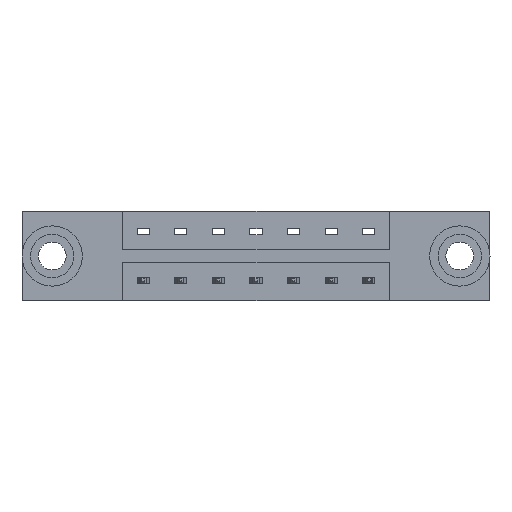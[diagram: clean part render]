
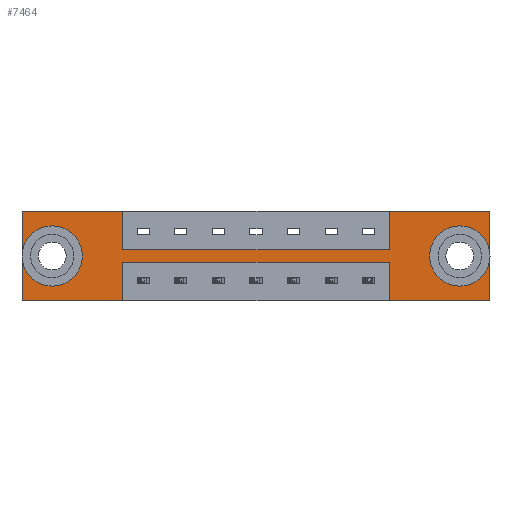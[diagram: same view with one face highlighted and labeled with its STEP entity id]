
A CAD part, front view. The second image highlights one B-rep face of the part: STEP entity #7464.
In plain terms, the highlighted planar face has unit normal (0, -1, 0).
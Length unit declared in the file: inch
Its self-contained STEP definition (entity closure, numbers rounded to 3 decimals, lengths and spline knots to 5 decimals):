
#50 = DIRECTION ( 'NONE',  ( 0., 0., 1. ) ) ;
#335 = CARTESIAN_POINT ( 'NONE',  ( 1.94, 0., 0. ) ) ;
#373 = ORIENTED_EDGE ( 'NONE', *, *, #9041, .F. ) ;
#390 = CARTESIAN_POINT ( 'NONE',  ( 0.4175, 0., -0.2115 ) ) ;
#518 = CARTESIAN_POINT ( 'NONE',  ( 1.5225, 0., -0.37 ) ) ;
#649 = AXIS2_PLACEMENT_3D ( 'NONE', #8227, #1374, #8664 ) ;
#770 = CARTESIAN_POINT ( 'NONE',  ( 1.5225, 0., -0.1585 ) ) ;
#817 = CIRCLE ( 'NONE', #2033, 0.078 ) ;
#856 = EDGE_CURVE ( 'NONE', #5274, #5009, #817, .T. ) ;
#886 = LINE ( 'NONE', #2596, #6320 ) ;
#990 = DIRECTION ( 'NONE',  ( 0., 0., -1. ) ) ;
#1005 = DIRECTION ( 'NONE',  ( 0., 0., 1. ) ) ;
#1165 = EDGE_CURVE ( 'NONE', #5626, #3667, #4683, .T. ) ;
#1167 = VERTEX_POINT ( 'NONE', #4730 ) ;
#1338 = VERTEX_POINT ( 'NONE', #4372 ) ;
#1363 = CARTESIAN_POINT ( 'NONE',  ( 1.815, 0., -0.185 ) ) ;
#1374 = DIRECTION ( 'NONE',  ( 0., 1., 0. ) ) ;
#1428 = DIRECTION ( 'NONE',  ( 0., 1., 0. ) ) ;
#1443 = VECTOR ( 'NONE', #990, 39.37008 ) ;
#1473 = VECTOR ( 'NONE', #3516, 39.37008 ) ;
#1480 = ORIENTED_EDGE ( 'NONE', *, *, #3855, .F. ) ;
#1493 = CARTESIAN_POINT ( 'NONE',  ( 1.94, 0., -0.37 ) ) ;
#1582 = CIRCLE ( 'NONE', #6945, 0.078 ) ;
#1645 = DIRECTION ( 'NONE',  ( 0., 0., 1. ) ) ;
#1690 = ORIENTED_EDGE ( 'NONE', *, *, #4533, .F. ) ;
#1694 = CARTESIAN_POINT ( 'NONE',  ( 0., 0., 0. ) ) ;
#1730 = FACE_BOUND ( 'NONE', #6455, .T. ) ;
#1777 = DIRECTION ( 'NONE',  ( -1., 0., 0. ) ) ;
#1828 = CARTESIAN_POINT ( 'NONE',  ( 0., 0., -0.37 ) ) ;
#1865 = DIRECTION ( 'NONE',  ( 0., -1., 0. ) ) ;
#1925 = DIRECTION ( 'NONE',  ( 1., 0., 0. ) ) ;
#1954 = EDGE_CURVE ( 'NONE', #8772, #3220, #3174, .T. ) ;
#2033 = AXIS2_PLACEMENT_3D ( 'NONE', #1363, #9316, #5022 ) ;
#2048 = VECTOR ( 'NONE', #1005, 39.37008 ) ;
#2087 = ORIENTED_EDGE ( 'NONE', *, *, #4001, .T. ) ;
#2151 = CARTESIAN_POINT ( 'NONE',  ( 0., 0., -0.37 ) ) ;
#2207 = CARTESIAN_POINT ( 'NONE',  ( 0.4175, 0., -0.2115 ) ) ;
#2354 = VECTOR ( 'NONE', #3242, 39.37008 ) ;
#2374 = CARTESIAN_POINT ( 'NONE',  ( 0.4175, 0., -0.1585 ) ) ;
#2454 = VERTEX_POINT ( 'NONE', #1493 ) ;
#2457 = CARTESIAN_POINT ( 'NONE',  ( 0.4175, 0., -0.37 ) ) ;
#2596 = CARTESIAN_POINT ( 'NONE',  ( 0., 0., 0. ) ) ;
#2638 = LINE ( 'NONE', #5570, #4500 ) ;
#2651 = LINE ( 'NONE', #335, #3475 ) ;
#2691 = ORIENTED_EDGE ( 'NONE', *, *, #1165, .F. ) ;
#2781 = CARTESIAN_POINT ( 'NONE',  ( 1.5225, 0., -0.1585 ) ) ;
#2901 = CARTESIAN_POINT ( 'NONE',  ( 1.5225, 0., 0. ) ) ;
#2927 = CARTESIAN_POINT ( 'NONE',  ( 0.125, 0., -0.185 ) ) ;
#2931 = LINE ( 'NONE', #2207, #5883 ) ;
#3144 = EDGE_CURVE ( 'NONE', #8902, #3191, #3716, .T. ) ;
#3174 = LINE ( 'NONE', #4558, #1443 ) ;
#3191 = VERTEX_POINT ( 'NONE', #6732 ) ;
#3220 = VERTEX_POINT ( 'NONE', #2374 ) ;
#3242 = DIRECTION ( 'NONE',  ( 0., 0., -1. ) ) ;
#3268 = CARTESIAN_POINT ( 'NONE',  ( 0., 0., -0.37 ) ) ;
#3282 = CARTESIAN_POINT ( 'NONE',  ( 0., 0., -0.37 ) ) ;
#3327 = ORIENTED_EDGE ( 'NONE', *, *, #7932, .F. ) ;
#3335 = DIRECTION ( 'NONE',  ( 0., 0., -1. ) ) ;
#3475 = VECTOR ( 'NONE', #5580, 39.37008 ) ;
#3516 = DIRECTION ( 'NONE',  ( 0., 0., 1. ) ) ;
#3526 = VERTEX_POINT ( 'NONE', #770 ) ;
#3595 = VECTOR ( 'NONE', #1777, 39.37008 ) ;
#3667 = VERTEX_POINT ( 'NONE', #2457 ) ;
#3716 = LINE ( 'NONE', #8886, #6214 ) ;
#3739 = ORIENTED_EDGE ( 'NONE', *, *, #856, .T. ) ;
#3813 = VERTEX_POINT ( 'NONE', #6146 ) ;
#3855 = EDGE_CURVE ( 'NONE', #3526, #4799, #9338, .T. ) ;
#3961 = DIRECTION ( 'NONE',  ( -1., 0., 0. ) ) ;
#4001 = EDGE_CURVE ( 'NONE', #1338, #3813, #5467, .T. ) ;
#4086 = ORIENTED_EDGE ( 'NONE', *, *, #8752, .F. ) ;
#4265 = ORIENTED_EDGE ( 'NONE', *, *, #8169, .T. ) ;
#4372 = CARTESIAN_POINT ( 'NONE',  ( 0.125, 0., -0.263 ) ) ;
#4458 = EDGE_LOOP ( 'NONE', ( #8244, #6761, #1690, #7707, #1480, #6316, #7811, #7162, #3327, #4086, #2691, #373 ) ) ;
#4500 = VECTOR ( 'NONE', #7780, 39.37008 ) ;
#4533 = EDGE_CURVE ( 'NONE', #6573, #2454, #2651, .T. ) ;
#4558 = CARTESIAN_POINT ( 'NONE',  ( 0.4175, 0., -0.1585 ) ) ;
#4666 = VECTOR ( 'NONE', #9408, 39.37008 ) ;
#4670 = FACE_OUTER_BOUND ( 'NONE', #4458, .T. ) ;
#4683 = LINE ( 'NONE', #390, #2354 ) ;
#4719 = CARTESIAN_POINT ( 'NONE',  ( 1.815, 0., -0.107 ) ) ;
#4730 = CARTESIAN_POINT ( 'NONE',  ( 0., 0., 0. ) ) ;
#4764 = LINE ( 'NONE', #3282, #9235 ) ;
#4799 = VERTEX_POINT ( 'NONE', #2901 ) ;
#4903 = CARTESIAN_POINT ( 'NONE',  ( 1.815, 0., -0.263 ) ) ;
#5009 = VERTEX_POINT ( 'NONE', #4719 ) ;
#5022 = DIRECTION ( 'NONE',  ( 0., 0., -1. ) ) ;
#5274 = VERTEX_POINT ( 'NONE', #4903 ) ;
#5287 = VERTEX_POINT ( 'NONE', #2151 ) ;
#5290 = CIRCLE ( 'NONE', #649, 0.078 ) ;
#5299 = DIRECTION ( 'NONE',  ( 0., 1., 0. ) ) ;
#5336 = LINE ( 'NONE', #3268, #3595 ) ;
#5467 = CIRCLE ( 'NONE', #6526, 0.078 ) ;
#5570 = CARTESIAN_POINT ( 'NONE',  ( 0.4175, 0., -0.1585 ) ) ;
#5578 = LINE ( 'NONE', #1694, #4666 ) ;
#5580 = DIRECTION ( 'NONE',  ( 0., 0., -1. ) ) ;
#5626 = VERTEX_POINT ( 'NONE', #8665 ) ;
#5883 = VECTOR ( 'NONE', #6717, 39.37008 ) ;
#6146 = CARTESIAN_POINT ( 'NONE',  ( 0.125, 0., -0.107 ) ) ;
#6147 = PLANE ( 'NONE',  #7263 ) ;
#6214 = VECTOR ( 'NONE', #50, 39.37008 ) ;
#6267 = EDGE_CURVE ( 'NONE', #4799, #6573, #886, .T. ) ;
#6316 = ORIENTED_EDGE ( 'NONE', *, *, #6402, .F. ) ;
#6320 = VECTOR ( 'NONE', #1925, 39.37008 ) ;
#6402 = EDGE_CURVE ( 'NONE', #3220, #3526, #2638, .T. ) ;
#6455 = EDGE_LOOP ( 'NONE', ( #8181, #2087 ) ) ;
#6526 = AXIS2_PLACEMENT_3D ( 'NONE', #2927, #1428, #8865 ) ;
#6573 = VERTEX_POINT ( 'NONE', #7243 ) ;
#6717 = DIRECTION ( 'NONE',  ( -1., 0., 0. ) ) ;
#6732 = CARTESIAN_POINT ( 'NONE',  ( 1.5225, 0., -0.2115 ) ) ;
#6761 = ORIENTED_EDGE ( 'NONE', *, *, #9155, .F. ) ;
#6807 = CARTESIAN_POINT ( 'NONE',  ( 0., 0., 0. ) ) ;
#6853 = LINE ( 'NONE', #6807, #2048 ) ;
#6945 = AXIS2_PLACEMENT_3D ( 'NONE', #8923, #5299, #1645 ) ;
#7123 = EDGE_CURVE ( 'NONE', #1167, #8772, #5578, .T. ) ;
#7162 = ORIENTED_EDGE ( 'NONE', *, *, #7123, .F. ) ;
#7243 = CARTESIAN_POINT ( 'NONE',  ( 1.94, 0., 0. ) ) ;
#7263 = AXIS2_PLACEMENT_3D ( 'NONE', #1828, #1865, #3335 ) ;
#7464 = ADVANCED_FACE ( 'NONE', ( #8298, #1730, #4670 ), #6147, .T. ) ;
#7678 = CARTESIAN_POINT ( 'NONE',  ( 0.4175, 0., 0. ) ) ;
#7707 = ORIENTED_EDGE ( 'NONE', *, *, #6267, .F. ) ;
#7780 = DIRECTION ( 'NONE',  ( 1., 0., 0. ) ) ;
#7811 = ORIENTED_EDGE ( 'NONE', *, *, #1954, .F. ) ;
#7932 = EDGE_CURVE ( 'NONE', #5287, #1167, #6853, .T. ) ;
#8169 = EDGE_CURVE ( 'NONE', #5009, #5274, #5290, .T. ) ;
#8181 = ORIENTED_EDGE ( 'NONE', *, *, #8677, .T. ) ;
#8227 = CARTESIAN_POINT ( 'NONE',  ( 1.815, 0., -0.185 ) ) ;
#8244 = ORIENTED_EDGE ( 'NONE', *, *, #3144, .F. ) ;
#8298 = FACE_BOUND ( 'NONE', #8978, .T. ) ;
#8664 = DIRECTION ( 'NONE',  ( 0., 0., -1. ) ) ;
#8665 = CARTESIAN_POINT ( 'NONE',  ( 0.4175, 0., -0.2115 ) ) ;
#8677 = EDGE_CURVE ( 'NONE', #3813, #1338, #1582, .T. ) ;
#8752 = EDGE_CURVE ( 'NONE', #3667, #5287, #4764, .T. ) ;
#8772 = VERTEX_POINT ( 'NONE', #7678 ) ;
#8865 = DIRECTION ( 'NONE',  ( 0., 0., 1. ) ) ;
#8886 = CARTESIAN_POINT ( 'NONE',  ( 1.5225, 0., -0.2115 ) ) ;
#8902 = VERTEX_POINT ( 'NONE', #518 ) ;
#8923 = CARTESIAN_POINT ( 'NONE',  ( 0.125, 0., -0.185 ) ) ;
#8978 = EDGE_LOOP ( 'NONE', ( #4265, #3739 ) ) ;
#9041 = EDGE_CURVE ( 'NONE', #3191, #5626, #2931, .T. ) ;
#9155 = EDGE_CURVE ( 'NONE', #2454, #8902, #5336, .T. ) ;
#9235 = VECTOR ( 'NONE', #3961, 39.37008 ) ;
#9316 = DIRECTION ( 'NONE',  ( 0., 1., 0. ) ) ;
#9338 = LINE ( 'NONE', #2781, #1473 ) ;
#9408 = DIRECTION ( 'NONE',  ( 1., 0., 0. ) ) ;
